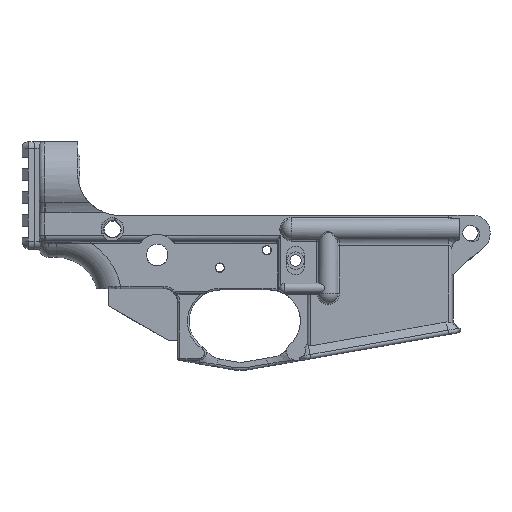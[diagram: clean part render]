
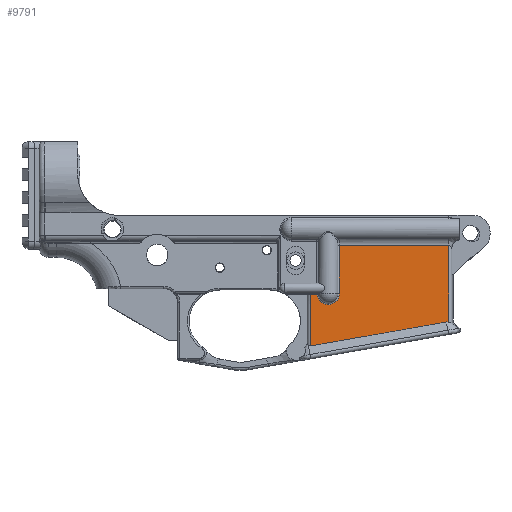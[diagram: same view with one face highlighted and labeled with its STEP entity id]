
A CAD part, left-side view. The second image highlights one B-rep face of the part: STEP entity #9791.
In plain terms, the highlighted planar face has unit normal (-1, 0, 0).
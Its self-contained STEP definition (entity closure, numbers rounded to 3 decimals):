
#302=PLANE('',#10747);
#833=LINE('',#20028,#1548);
#834=LINE('',#20030,#1549);
#835=LINE('',#20033,#1550);
#836=LINE('',#20052,#1551);
#990=LINE('',#21774,#1705);
#991=LINE('',#21775,#1706);
#1548=VECTOR('',#12658,62.909);
#1549=VECTOR('',#12661,23.276);
#1550=VECTOR('',#12664,2.864);
#1551=VECTOR('',#12673,21.861);
#1705=VECTOR('',#13187,35.127);
#1706=VECTOR('',#13188,49.812);
#2574=FACE_OUTER_BOUND('',#3155,.T.);
#3155=EDGE_LOOP('',(#8744,#8745,#8746,#8747,#8748,#8749,#8750,#8751));
#3467=B_SPLINE_CURVE_WITH_KNOTS('',3,(#21766,#21767,#21768,#21769,#21770,
#21771),.UNSPECIFIED.,.F.,.F.,(4,2,4),(-0.114,-0.051,
0.),.UNSPECIFIED.);
#3797=CIRCLE('',#10565,5.168);
#4371=VERTEX_POINT('',#17759);
#4566=VERTEX_POINT('',#20024);
#4567=VERTEX_POINT('',#20026);
#4568=VERTEX_POINT('',#20032);
#4569=VERTEX_POINT('',#20047);
#4570=VERTEX_POINT('',#20051);
#4764=VERTEX_POINT('',#21755);
#4765=VERTEX_POINT('',#21773);
#5850=EDGE_CURVE('',#4566,#4567,#833,.T.);
#5851=EDGE_CURVE('',#4566,#4371,#834,.T.);
#5852=EDGE_CURVE('',#4568,#4371,#835,.T.);
#5854=EDGE_CURVE('',#4568,#4569,#3797,.T.);
#5856=EDGE_CURVE('',#4570,#4569,#836,.T.);
#6160=EDGE_CURVE('',#4567,#4764,#3467,.T.);
#6161=EDGE_CURVE('',#4764,#4765,#990,.T.);
#6162=EDGE_CURVE('',#4765,#4570,#991,.T.);
#8744=ORIENTED_EDGE('',*,*,#6160,.T.);
#8745=ORIENTED_EDGE('',*,*,#6161,.T.);
#8746=ORIENTED_EDGE('',*,*,#6162,.T.);
#8747=ORIENTED_EDGE('',*,*,#5856,.T.);
#8748=ORIENTED_EDGE('',*,*,#5854,.F.);
#8749=ORIENTED_EDGE('',*,*,#5852,.T.);
#8750=ORIENTED_EDGE('',*,*,#5851,.F.);
#8751=ORIENTED_EDGE('',*,*,#5850,.T.);
#9791=ADVANCED_FACE('',(#2574),#302,.T.);
#10565=AXIS2_PLACEMENT_3D('',#20048,#12667,#12668);
#10747=AXIS2_PLACEMENT_3D('',#21772,#13185,#13186);
#12658=DIRECTION('',(0.,-0.985,0.174));
#12661=DIRECTION('',(0.,0.,1.));
#12664=DIRECTION('',(0.,1.,0.));
#12667=DIRECTION('center_axis',(-1.,0.,0.));
#12668=DIRECTION('ref_axis',(0.,-1.,0.));
#12673=DIRECTION('',(0.,0.,-1.));
#13185=DIRECTION('center_axis',(-1.,0.,0.));
#13186=DIRECTION('ref_axis',(0.,0.,
-1.));
#13187=DIRECTION('',(0.,0.,1.));
#13188=DIRECTION('',(0.,1.,0.));
#17759=CARTESIAN_POINT('',(-0.558,471.069,131.711));
#20024=CARTESIAN_POINT('',(-0.558,471.069,108.435));
#20026=CARTESIAN_POINT('',(-0.558,409.116,119.359));
#20028=CARTESIAN_POINT('',(-0.558,471.069,108.435));
#20030=CARTESIAN_POINT('',(-0.558,471.069,108.435));
#20032=CARTESIAN_POINT('',(-0.558,468.205,131.711));
#20033=CARTESIAN_POINT('',(-0.558,468.205,131.711));
#20047=CARTESIAN_POINT('',(-0.558,457.926,132.473));
#20048=CARTESIAN_POINT('Origin',(-0.558,463.094,132.473));
#20051=CARTESIAN_POINT('',(-0.558,457.926,154.335));
#20052=CARTESIAN_POINT('',(-0.558,457.926,154.335));
#21755=CARTESIAN_POINT('',(-0.558,408.113,119.207));
#21766=CARTESIAN_POINT('Ctrl Pts',(-0.558,409.116,119.359));
#21767=CARTESIAN_POINT('Ctrl Pts',(-0.558,408.979,119.383));
#21768=CARTESIAN_POINT('Ctrl Pts',(-0.558,408.813,
119.39));
#21769=CARTESIAN_POINT('Ctrl Pts',(-0.558,408.438,
119.325));
#21770=CARTESIAN_POINT('Ctrl Pts',(-0.558,408.272,
119.271));
#21771=CARTESIAN_POINT('Ctrl Pts',(-0.558,408.113,
119.207));
#21772=CARTESIAN_POINT('Origin',(-0.558,439.591,108.159));
#21773=CARTESIAN_POINT('',(-0.558,408.113,154.335));
#21774=CARTESIAN_POINT('',(-0.558,408.113,119.207));
#21775=CARTESIAN_POINT('',(-0.558,408.113,154.335));
